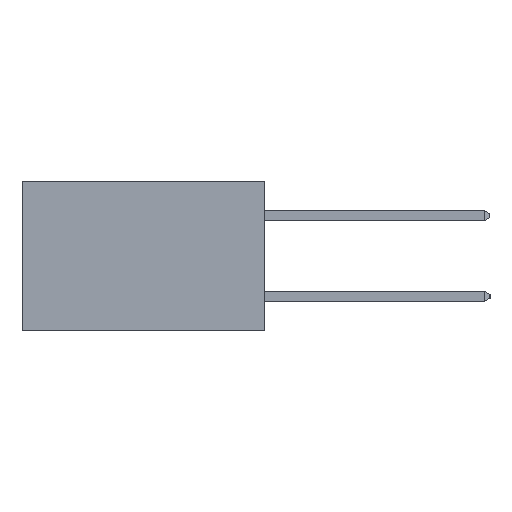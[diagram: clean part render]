
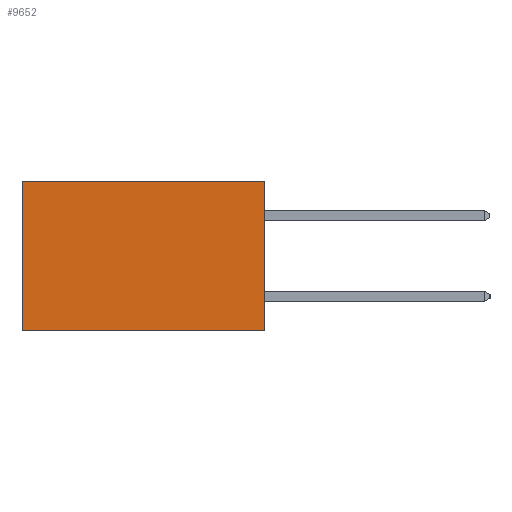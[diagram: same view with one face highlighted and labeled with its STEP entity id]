
A CAD part, left-side view. The second image highlights one B-rep face of the part: STEP entity #9652.
In plain terms, the highlighted planar face has unit normal (-1, 0, 0).
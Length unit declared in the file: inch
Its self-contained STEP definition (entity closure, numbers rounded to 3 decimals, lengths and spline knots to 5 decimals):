
#1383 = DIRECTION ( 'NONE',  ( 0., 0., -1. ) ) ;
#1905 = CARTESIAN_POINT ( 'NONE',  ( 0.2615, 0.6, -0.37 ) ) ;
#2957 = EDGE_CURVE ( 'NONE', #9136, #10591, #8085, .T. ) ;
#3006 = ORIENTED_EDGE ( 'NONE', *, *, #6937, .F. ) ;
#3242 = ORIENTED_EDGE ( 'NONE', *, *, #2957, .T. ) ;
#3357 = CARTESIAN_POINT ( 'NONE',  ( 0.2615, 0., -0.37 ) ) ;
#3602 = EDGE_CURVE ( 'NONE', #12271, #10591, #8524, .T. ) ;
#4664 = CARTESIAN_POINT ( 'NONE',  ( 0.2615, 0.6, 0. ) ) ;
#4733 = FACE_OUTER_BOUND ( 'NONE', #11731, .T. ) ;
#5243 = LINE ( 'NONE', #8518, #9934 ) ;
#5269 = ORIENTED_EDGE ( 'NONE', *, *, #6292, .T. ) ;
#5345 = PLANE ( 'NONE',  #5893 ) ;
#5893 = AXIS2_PLACEMENT_3D ( 'NONE', #3357, #7375, #1383 ) ;
#6292 = EDGE_CURVE ( 'NONE', #10428, #9136, #12231, .T. ) ;
#6517 = DIRECTION ( 'NONE',  ( 0., 0., -1. ) ) ;
#6542 = ORIENTED_EDGE ( 'NONE', *, *, #3602, .F. ) ;
#6600 = DIRECTION ( 'NONE',  ( 0., 0., -1. ) ) ;
#6937 = EDGE_CURVE ( 'NONE', #10428, #12271, #5243, .T. ) ;
#7375 = DIRECTION ( 'NONE',  ( 1., 0., 0. ) ) ;
#7663 = CARTESIAN_POINT ( 'NONE',  ( 0.2615, 0., 0. ) ) ;
#7762 = VECTOR ( 'NONE', #6600, 39.37008 ) ;
#7895 = CARTESIAN_POINT ( 'NONE',  ( 0.2615, 0.6, -0.37 ) ) ;
#8085 = LINE ( 'NONE', #7895, #7762 ) ;
#8518 = CARTESIAN_POINT ( 'NONE',  ( 0.2615, 0., -0.37 ) ) ;
#8524 = LINE ( 'NONE', #11223, #10885 ) ;
#9136 = VERTEX_POINT ( 'NONE', #4664 ) ;
#9652 = ADVANCED_FACE ( 'NONE', ( #4733 ), #5345, .F. ) ;
#9858 = DIRECTION ( 'NONE',  ( 0., 1., 0. ) ) ;
#9886 = CARTESIAN_POINT ( 'NONE',  ( 0.2615, 0., 0. ) ) ;
#9934 = VECTOR ( 'NONE', #6517, 39.37008 ) ;
#10428 = VERTEX_POINT ( 'NONE', #7663 ) ;
#10591 = VERTEX_POINT ( 'NONE', #1905 ) ;
#10885 = VECTOR ( 'NONE', #11060, 39.37008 ) ;
#11060 = DIRECTION ( 'NONE',  ( 0., 1., 0. ) ) ;
#11223 = CARTESIAN_POINT ( 'NONE',  ( 0.2615, 0., -0.37 ) ) ;
#11731 = EDGE_LOOP ( 'NONE', ( #3242, #6542, #3006, #5269 ) ) ;
#12231 = LINE ( 'NONE', #9886, #12512 ) ;
#12271 = VERTEX_POINT ( 'NONE', #12363 ) ;
#12363 = CARTESIAN_POINT ( 'NONE',  ( 0.2615, 0., -0.37 ) ) ;
#12512 = VECTOR ( 'NONE', #9858, 39.37008 ) ;
